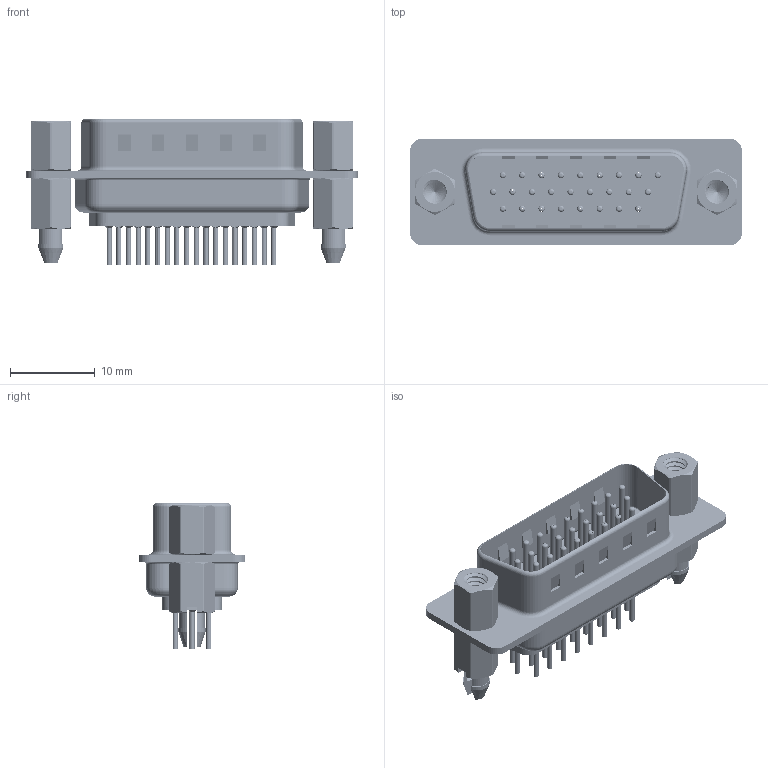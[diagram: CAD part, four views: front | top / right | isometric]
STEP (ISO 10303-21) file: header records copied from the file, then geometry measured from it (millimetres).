
FILE_DESCRIPTION (( 'STEP AP203' ), '1' );
FILE_NAME ('637-026-630-247.STEP', '2020-07-18T01:19:49', ( '' ), ( '' ), 'SwSTEP 2.0', 'SolidWorks 2020', '' );
FILE_SCHEMA (( 'CONFIG_CONTROL_DESIGN' ));
Length unit declared in the file: millimetre
Products named in the file (9): 637 Contact Row 1_30; 637 Shell Rear_26 Contacts; 637 Contact Row 3_30; 637 Contact Row 2_30; 637 4-40 Hex Standoff; 637 4-40 Threaded Boardlock_LP; 637 Housing_26 Contacts; 637 Shell Front_26 Contacts; 637-026-630-247
Assembly tree (33 placements, depth 2):
  637-026-630-247
    637 Housing_26 Contacts
    637 Shell Front_26 Contacts
    637 Shell Rear_26 Contacts
    637 Contact Row 1_30  x9
    637 Contact Row 2_30  x9
    637 Contact Row 3_30  x8
    637 4-40 Hex Standoff  x2
    637 4-40 Threaded Boardlock_LP  x2
Bounding box: 39.2 x 12.6 x 17.25 mm (x, y, z)
Volume: 2153.9 mm3; surface area: 7461.3 mm2
Topology: 33 solids, 33 shells, 3140 faces, 8327 edges, 5158 vertices
Faces by surface type: cylinder 1199, plane 817, torus 804, cone 302, bspline 18
Entity records: 33280 total; most frequent: CARTESIAN_POINT 9744, DIRECTION 4819, ORIENTED_EDGE 4498, EDGE_CURVE 2249, AXIS2_PLACEMENT_3D 1935, VERTEX_POINT 1436, EDGE_LOOP 1039, CIRCLE 1017
